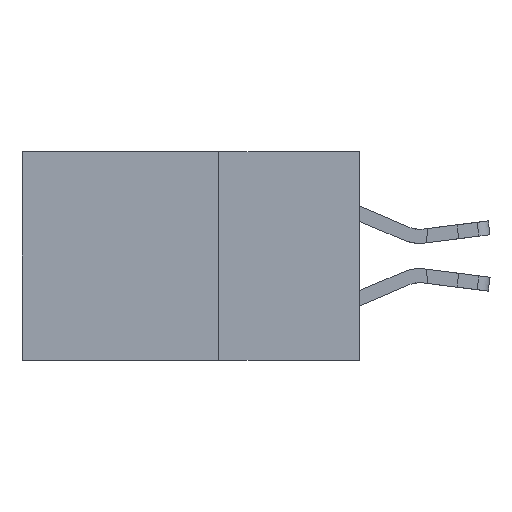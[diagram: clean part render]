
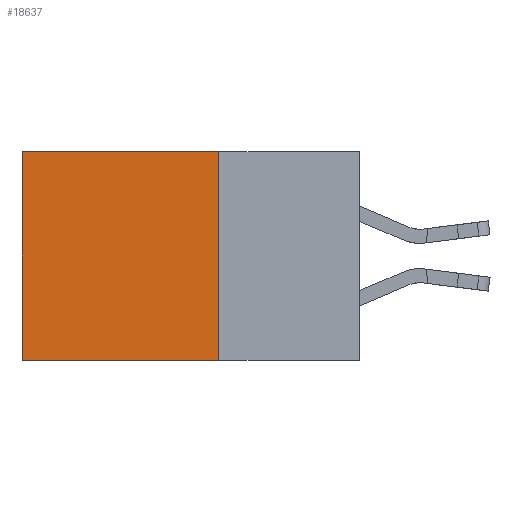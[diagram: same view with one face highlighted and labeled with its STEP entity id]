
A CAD part, left-side view. The second image highlights one B-rep face of the part: STEP entity #18637.
In plain terms, the highlighted planar face has unit normal (-1, 0, 0).
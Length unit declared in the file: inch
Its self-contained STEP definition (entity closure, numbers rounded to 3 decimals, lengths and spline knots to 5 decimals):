
#418 = ORIENTED_EDGE ( 'NONE', *, *, #4165, .F. ) ;
#763 = CARTESIAN_POINT ( 'NONE',  ( 0.2875, 0.6, -0.37 ) ) ;
#996 = VECTOR ( 'NONE', #12014, 39.37008 ) ;
#3648 = CARTESIAN_POINT ( 'NONE',  ( 0.2875, 0.25, -0.37 ) ) ;
#4165 = EDGE_CURVE ( 'NONE', #19625, #29012, #20601, .T. ) ;
#5224 = CARTESIAN_POINT ( 'NONE',  ( 0.2875, 0.25, 0. ) ) ;
#6045 = EDGE_CURVE ( 'NONE', #19625, #24182, #24683, .T. ) ;
#7325 = EDGE_LOOP ( 'NONE', ( #17629, #17659, #418, #14959 ) ) ;
#8175 = LINE ( 'NONE', #3648, #13529 ) ;
#11111 = CARTESIAN_POINT ( 'NONE',  ( 0.2875, 0.25, -0.37 ) ) ;
#11270 = CARTESIAN_POINT ( 'NONE',  ( 0.2875, 0.6, 0. ) ) ;
#11547 = CARTESIAN_POINT ( 'NONE',  ( 0.2875, 0.25, 0. ) ) ;
#11995 = DIRECTION ( 'NONE',  ( 0., 0., -1. ) ) ;
#12014 = DIRECTION ( 'NONE',  ( 0., 0., -1. ) ) ;
#12534 = CARTESIAN_POINT ( 'NONE',  ( 0.2875, 0.25, 0. ) ) ;
#12579 = EDGE_CURVE ( 'NONE', #24182, #26894, #23483, .T. ) ;
#12777 = DIRECTION ( 'NONE',  ( 0., 1., 0. ) ) ;
#13529 = VECTOR ( 'NONE', #12777, 39.37008 ) ;
#14959 = ORIENTED_EDGE ( 'NONE', *, *, #6045, .T. ) ;
#15459 = VECTOR ( 'NONE', #26106, 39.37008 ) ;
#17629 = ORIENTED_EDGE ( 'NONE', *, *, #12579, .T. ) ;
#17659 = ORIENTED_EDGE ( 'NONE', *, *, #21234, .F. ) ;
#18084 = CARTESIAN_POINT ( 'NONE',  ( 0.2875, 0.6, 0. ) ) ;
#18473 = VECTOR ( 'NONE', #11995, 39.37008 ) ;
#18637 = ADVANCED_FACE ( 'NONE', ( #19915 ), #26063, .F. ) ;
#19625 = VERTEX_POINT ( 'NONE', #11547 ) ;
#19915 = FACE_OUTER_BOUND ( 'NONE', #7325, .T. ) ;
#20601 = LINE ( 'NONE', #5224, #996 ) ;
#21234 = EDGE_CURVE ( 'NONE', #29012, #26894, #8175, .T. ) ;
#22218 = DIRECTION ( 'NONE',  ( 1., 0., 0. ) ) ;
#23483 = LINE ( 'NONE', #11270, #18473 ) ;
#24182 = VERTEX_POINT ( 'NONE', #18084 ) ;
#24683 = LINE ( 'NONE', #25922, #15459 ) ;
#25922 = CARTESIAN_POINT ( 'NONE',  ( 0.2875, 0.25, 0. ) ) ;
#26063 = PLANE ( 'NONE',  #29144 ) ;
#26106 = DIRECTION ( 'NONE',  ( 0., 1., 0. ) ) ;
#26894 = VERTEX_POINT ( 'NONE', #763 ) ;
#28833 = DIRECTION ( 'NONE',  ( 0., 0., -1. ) ) ;
#29012 = VERTEX_POINT ( 'NONE', #11111 ) ;
#29144 = AXIS2_PLACEMENT_3D ( 'NONE', #12534, #22218, #28833 ) ;
